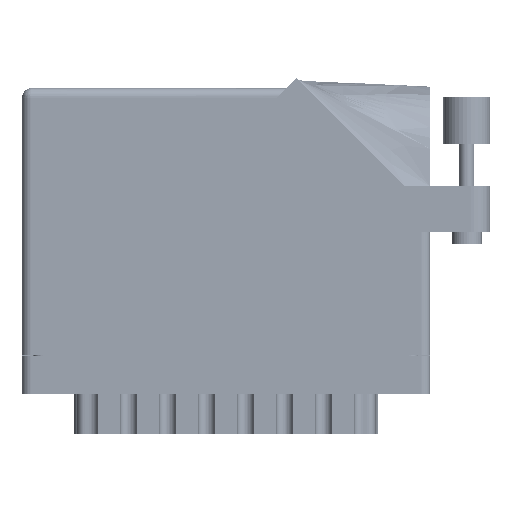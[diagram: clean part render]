
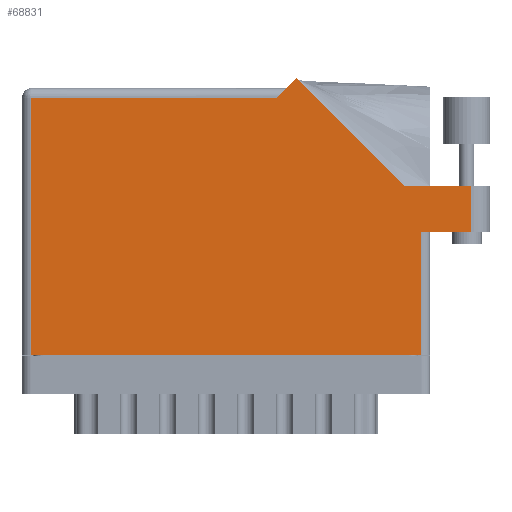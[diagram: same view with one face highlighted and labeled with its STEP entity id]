
A CAD part, front view. The second image highlights one B-rep face of the part: STEP entity #68831.
In plain terms, the highlighted face is planar.
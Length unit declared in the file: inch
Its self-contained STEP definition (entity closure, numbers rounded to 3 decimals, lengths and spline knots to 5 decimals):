
#385 = VECTOR ( 'NONE', #39503, 39.37008 ) ;
#992 = CARTESIAN_POINT ( 'NONE',  ( 2.656, 0.815, 0. ) ) ;
#1761 = EDGE_CURVE ( 'NONE', #11305, #57198, #22135, .T. ) ;
#2795 = CARTESIAN_POINT ( 'NONE',  ( 2.993, 0.815, 0. ) ) ;
#3378 = LINE ( 'NONE', #46824, #8946 ) ;
#3835 = ORIENTED_EDGE ( 'NONE', *, *, #26873, .T. ) ;
#4191 = ORIENTED_EDGE ( 'NONE', *, *, #26764, .T. ) ;
#6068 = LINE ( 'NONE', #7215, #70753 ) ;
#6447 = EDGE_CURVE ( 'NONE', #53889, #67687, #56306, .T. ) ;
#7215 = CARTESIAN_POINT ( 'NONE',  ( 1.758, 1.775, 0. ) ) ;
#8013 = FACE_OUTER_BOUND ( 'NONE', #56319, .T. ) ;
#8946 = VECTOR ( 'NONE', #29026, 39.37008 ) ;
#9381 = VECTOR ( 'NONE', #74622, 39.37008 ) ;
#9524 = CARTESIAN_POINT ( 'NONE',  ( 0.062, 1.713, 0. ) ) ;
#10073 = VERTEX_POINT ( 'NONE', #25636 ) ;
#11305 = VERTEX_POINT ( 'NONE', #9524 ) ;
#12401 = CARTESIAN_POINT ( 'NONE',  ( 2.656, 0., 0. ) ) ;
#16281 = CARTESIAN_POINT ( 'NONE',  ( 2.993, 1.122, 0. ) ) ;
#16722 = CARTESIAN_POINT ( 'NONE',  ( 2.55242, 1.122, 0. ) ) ;
#17872 = EDGE_CURVE ( 'NONE', #67687, #66734, #25167, .T. ) ;
#18354 = VERTEX_POINT ( 'NONE', #16722 ) ;
#18417 = VECTOR ( 'NONE', #23872, 39.37008 ) ;
#19735 = PLANE ( 'NONE',  #34587 ) ;
#19776 = LINE ( 'NONE', #62204, #52111 ) ;
#19897 = LINE ( 'NONE', #74796, #385 ) ;
#20075 = CARTESIAN_POINT ( 'NONE',  ( 0.062, 0., 0. ) ) ;
#22135 = LINE ( 'NONE', #20075, #75625 ) ;
#23542 = ORIENTED_EDGE ( 'NONE', *, *, #71641, .T. ) ;
#23872 = DIRECTION ( 'NONE',  ( 1., 0., 0. ) ) ;
#24639 = DIRECTION ( 'NONE',  ( -0.707, -0.707, 0. ) ) ;
#24922 = CARTESIAN_POINT ( 'NONE',  ( 0., 1.775, 0. ) ) ;
#25167 = LINE ( 'NONE', #16281, #9381 ) ;
#25636 = CARTESIAN_POINT ( 'NONE',  ( 1.696, 1.713, 0. ) ) ;
#26764 = EDGE_CURVE ( 'NONE', #10073, #11305, #19897, .T. ) ;
#26873 = EDGE_CURVE ( 'NONE', #57198, #56614, #29106, .T. ) ;
#29026 = DIRECTION ( 'NONE',  ( 0., 1., 0. ) ) ;
#29106 = LINE ( 'NONE', #64919, #60478 ) ;
#34587 = AXIS2_PLACEMENT_3D ( 'NONE', #24922, #43502, #55331 ) ;
#37637 = ORIENTED_EDGE ( 'NONE', *, *, #51736, .T. ) ;
#38174 = DIRECTION ( 'NONE',  ( 0., -1., 0. ) ) ;
#38309 = VECTOR ( 'NONE', #75136, 39.37008 ) ;
#39503 = DIRECTION ( 'NONE',  ( -1., 0., 0. ) ) ;
#42384 = EDGE_CURVE ( 'NONE', #66734, #18354, #71454, .T. ) ;
#43502 = DIRECTION ( 'NONE',  ( 0., 0., -1. ) ) ;
#46303 = EDGE_CURVE ( 'NONE', #52573, #10073, #6068, .T. ) ;
#46824 = CARTESIAN_POINT ( 'NONE',  ( 2.656, 0.815, 0. ) ) ;
#47785 = ORIENTED_EDGE ( 'NONE', *, *, #6447, .T. ) ;
#51736 = EDGE_CURVE ( 'NONE', #56614, #53889, #3378, .T. ) ;
#52111 = VECTOR ( 'NONE', #68836, 39.37008 ) ;
#52573 = VERTEX_POINT ( 'NONE', #60350 ) ;
#52986 = ORIENTED_EDGE ( 'NONE', *, *, #17872, .T. ) ;
#53138 = ORIENTED_EDGE ( 'NONE', *, *, #42384, .T. ) ;
#53527 = ORIENTED_EDGE ( 'NONE', *, *, #46303, .T. ) ;
#53889 = VERTEX_POINT ( 'NONE', #992 ) ;
#55331 = DIRECTION ( 'NONE',  ( -1., 0., 0. ) ) ;
#56306 = LINE ( 'NONE', #59218, #18417 ) ;
#56319 = EDGE_LOOP ( 'NONE', ( #47785, #52986, #53138, #23542, #53527, #4191, #60739, #3835, #37637 ) ) ;
#56614 = VERTEX_POINT ( 'NONE', #12401 ) ;
#57198 = VERTEX_POINT ( 'NONE', #60424 ) ;
#59038 = DIRECTION ( 'NONE',  ( 1., 0., 0. ) ) ;
#59218 = CARTESIAN_POINT ( 'NONE',  ( 2.718, 0.815, 0. ) ) ;
#60350 = CARTESIAN_POINT ( 'NONE',  ( 1.82871, 1.84571, 0. ) ) ;
#60424 = CARTESIAN_POINT ( 'NONE',  ( 0.062, 0., 0. ) ) ;
#60478 = VECTOR ( 'NONE', #59038, 39.37008 ) ;
#60739 = ORIENTED_EDGE ( 'NONE', *, *, #1761, .T. ) ;
#62204 = CARTESIAN_POINT ( 'NONE',  ( 2.55242, 1.122, 0. ) ) ;
#64919 = CARTESIAN_POINT ( 'NONE',  ( 0., 0., 0. ) ) ;
#66734 = VERTEX_POINT ( 'NONE', #67100 ) ;
#67100 = CARTESIAN_POINT ( 'NONE',  ( 2.993, 1.122, 0. ) ) ;
#67687 = VERTEX_POINT ( 'NONE', #2795 ) ;
#68831 = ADVANCED_FACE ( 'NONE', ( #8013 ), #19735, .F. ) ;
#68836 = DIRECTION ( 'NONE',  ( -0.707, 0.707, 0. ) ) ;
#70753 = VECTOR ( 'NONE', #24639, 39.37008 ) ;
#71454 = LINE ( 'NONE', #74881, #38309 ) ;
#71641 = EDGE_CURVE ( 'NONE', #18354, #52573, #19776, .T. ) ;
#74622 = DIRECTION ( 'NONE',  ( 0., 1., 0. ) ) ;
#74796 = CARTESIAN_POINT ( 'NONE',  ( 0., 1.713, 0. ) ) ;
#74881 = CARTESIAN_POINT ( 'NONE',  ( 3.118, 1.122, 0. ) ) ;
#75136 = DIRECTION ( 'NONE',  ( -1., 0., 0. ) ) ;
#75625 = VECTOR ( 'NONE', #38174, 39.37008 ) ;
